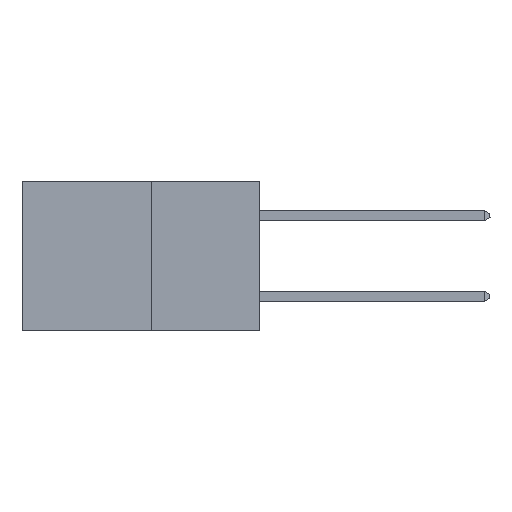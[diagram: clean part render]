
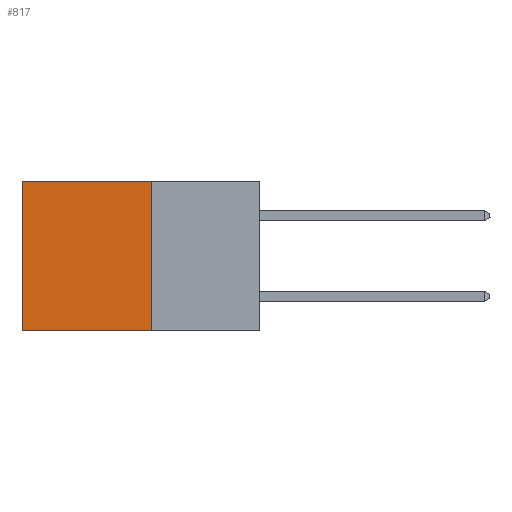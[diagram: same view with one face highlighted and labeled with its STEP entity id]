
A CAD part, left-side view. The second image highlights one B-rep face of the part: STEP entity #817.
In plain terms, the highlighted planar face has unit normal (-1, 0, 0).
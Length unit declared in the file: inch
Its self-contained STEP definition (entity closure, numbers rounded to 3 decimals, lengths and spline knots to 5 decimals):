
#817 = ADVANCED_FACE ( 'NONE', ( #18705 ), #20875, .F. ) ;
#890 = VERTEX_POINT ( 'NONE', #14772 ) ;
#1607 = AXIS2_PLACEMENT_3D ( 'NONE', #21096, #20674, #20370 ) ;
#2130 = EDGE_CURVE ( 'NONE', #890, #9322, #32537, .T. ) ;
#4764 = VERTEX_POINT ( 'NONE', #26392 ) ;
#5650 = CARTESIAN_POINT ( 'NONE',  ( 0.277, 0.27, 0. ) ) ;
#7542 = DIRECTION ( 'NONE',  ( 0., 1., 0. ) ) ;
#7713 = ORIENTED_EDGE ( 'NONE', *, *, #33731, .T. ) ;
#9322 = VERTEX_POINT ( 'NONE', #25273 ) ;
#10594 = VECTOR ( 'NONE', #26608, 39.37008 ) ;
#11328 = EDGE_LOOP ( 'NONE', ( #33945, #21381, #22062, #7713 ) ) ;
#12820 = CARTESIAN_POINT ( 'NONE',  ( 0.277, 0.27, -0.37 ) ) ;
#14772 = CARTESIAN_POINT ( 'NONE',  ( 0.277, 0.27, 0. ) ) ;
#15826 = CARTESIAN_POINT ( 'NONE',  ( 0.277, 0.59, -0.37 ) ) ;
#17595 = VECTOR ( 'NONE', #7542, 39.37008 ) ;
#18705 = FACE_OUTER_BOUND ( 'NONE', #11328, .T. ) ;
#20370 = DIRECTION ( 'NONE',  ( 0., 0., -1. ) ) ;
#20674 = DIRECTION ( 'NONE',  ( 1., 0., 0. ) ) ;
#20875 = PLANE ( 'NONE',  #1607 ) ;
#21072 = CARTESIAN_POINT ( 'NONE',  ( 0.277, 0.59, 0. ) ) ;
#21096 = CARTESIAN_POINT ( 'NONE',  ( 0.277, 0.27, -0.37 ) ) ;
#21381 = ORIENTED_EDGE ( 'NONE', *, *, #23883, .F. ) ;
#22062 = ORIENTED_EDGE ( 'NONE', *, *, #2130, .F. ) ;
#22122 = EDGE_CURVE ( 'NONE', #27539, #4764, #24841, .T. ) ;
#23883 = EDGE_CURVE ( 'NONE', #9322, #4764, #24709, .T. ) ;
#24709 = LINE ( 'NONE', #12820, #17595 ) ;
#24841 = LINE ( 'NONE', #15826, #10594 ) ;
#25273 = CARTESIAN_POINT ( 'NONE',  ( 0.277, 0.27, -0.37 ) ) ;
#25358 = VECTOR ( 'NONE', #34462, 39.37008 ) ;
#25899 = VECTOR ( 'NONE', #32428, 39.37008 ) ;
#26392 = CARTESIAN_POINT ( 'NONE',  ( 0.277, 0.59, -0.37 ) ) ;
#26608 = DIRECTION ( 'NONE',  ( 0., 0., -1. ) ) ;
#26744 = LINE ( 'NONE', #5650, #25899 ) ;
#27539 = VERTEX_POINT ( 'NONE', #21072 ) ;
#32338 = CARTESIAN_POINT ( 'NONE',  ( 0.277, 0.27, -0.37 ) ) ;
#32428 = DIRECTION ( 'NONE',  ( 0., 1., 0. ) ) ;
#32537 = LINE ( 'NONE', #32338, #25358 ) ;
#33731 = EDGE_CURVE ( 'NONE', #890, #27539, #26744, .T. ) ;
#33945 = ORIENTED_EDGE ( 'NONE', *, *, #22122, .T. ) ;
#34462 = DIRECTION ( 'NONE',  ( 0., 0., -1. ) ) ;
